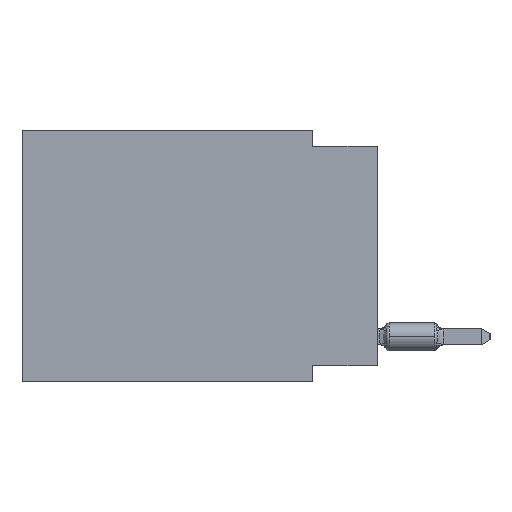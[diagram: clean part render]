
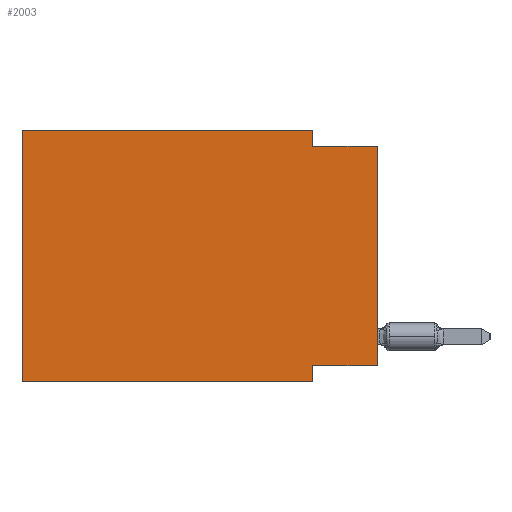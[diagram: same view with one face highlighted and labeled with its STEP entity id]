
A CAD part, left-side view. The second image highlights one B-rep face of the part: STEP entity #2003.
In plain terms, the highlighted planar face has unit normal (-1, 0, 0).
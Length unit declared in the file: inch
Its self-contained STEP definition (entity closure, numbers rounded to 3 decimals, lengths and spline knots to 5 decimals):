
#384 = PLANE ( 'NONE',  #32318 ) ;
#400 = LINE ( 'NONE', #17830, #42309 ) ;
#711 = VERTEX_POINT ( 'NONE', #39553 ) ;
#2003 = ADVANCED_FACE ( 'NONE', ( #34695 ), #384, .F. ) ;
#2099 = ORIENTED_EDGE ( 'NONE', *, *, #7044, .F. ) ;
#4460 = LINE ( 'NONE', #39086, #16757 ) ;
#5492 = CARTESIAN_POINT ( 'NONE',  ( 0., 0., -0.025 ) ) ;
#6367 = CARTESIAN_POINT ( 'NONE',  ( 0., 0.1, -0.39 ) ) ;
#7044 = EDGE_CURVE ( 'NONE', #51285, #8439, #31570, .T. ) ;
#8439 = VERTEX_POINT ( 'NONE', #15037 ) ;
#9232 = DIRECTION ( 'NONE',  ( 0., -1., 0. ) ) ;
#9585 = ORIENTED_EDGE ( 'NONE', *, *, #18488, .T. ) ;
#10608 = LINE ( 'NONE', #5492, #35398 ) ;
#12767 = LINE ( 'NONE', #21637, #32019 ) ;
#13049 = DIRECTION ( 'NONE',  ( 0., 1., 0. ) ) ;
#15013 = CARTESIAN_POINT ( 'NONE',  ( 0., 0.55, 0. ) ) ;
#15037 = CARTESIAN_POINT ( 'NONE',  ( 0., 0.1, -0.025 ) ) ;
#15389 = VERTEX_POINT ( 'NONE', #48682 ) ;
#16171 = VERTEX_POINT ( 'NONE', #43898 ) ;
#16757 = VECTOR ( 'NONE', #47970, 39.37008 ) ;
#17830 = CARTESIAN_POINT ( 'NONE',  ( 0., 0.55, -0.39 ) ) ;
#18095 = DIRECTION ( 'NONE',  ( 1., 0., 0. ) ) ;
#18488 = EDGE_CURVE ( 'NONE', #51190, #44938, #400, .T. ) ;
#18976 = EDGE_CURVE ( 'NONE', #711, #16171, #4460, .T. ) ;
#19512 = LINE ( 'NONE', #6367, #38303 ) ;
#21273 = ORIENTED_EDGE ( 'NONE', *, *, #32493, .F. ) ;
#21616 = CARTESIAN_POINT ( 'NONE',  ( 0., 0.55, 0. ) ) ;
#21637 = CARTESIAN_POINT ( 'NONE',  ( 0., 0., -0.365 ) ) ;
#21758 = EDGE_CURVE ( 'NONE', #51190, #42476, #39363, .T. ) ;
#23003 = DIRECTION ( 'NONE',  ( 0., 0., -1. ) ) ;
#23821 = DIRECTION ( 'NONE',  ( 0., 0., -1. ) ) ;
#25809 = CARTESIAN_POINT ( 'NONE',  ( 0., 0.55, 0. ) ) ;
#28436 = LINE ( 'NONE', #15013, #45415 ) ;
#29611 = ORIENTED_EDGE ( 'NONE', *, *, #18976, .T. ) ;
#31570 = LINE ( 'NONE', #49621, #54193 ) ;
#32019 = VECTOR ( 'NONE', #13049, 39.37008 ) ;
#32166 = ORIENTED_EDGE ( 'NONE', *, *, #43776, .F. ) ;
#32318 = AXIS2_PLACEMENT_3D ( 'NONE', #25809, #18095, #43866 ) ;
#32493 = EDGE_CURVE ( 'NONE', #15389, #44938, #19512, .T. ) ;
#34695 = FACE_OUTER_BOUND ( 'NONE', #53881, .T. ) ;
#35398 = VECTOR ( 'NONE', #54436, 39.37008 ) ;
#36012 = CARTESIAN_POINT ( 'NONE',  ( 0., 0.55, 0. ) ) ;
#36188 = DIRECTION ( 'NONE',  ( 0., -1., 0. ) ) ;
#36712 = CARTESIAN_POINT ( 'NONE',  ( 0., 0.55, -0.39 ) ) ;
#38303 = VECTOR ( 'NONE', #23821, 39.37008 ) ;
#39086 = CARTESIAN_POINT ( 'NONE',  ( 0., 0., 0. ) ) ;
#39363 = LINE ( 'NONE', #21616, #54457 ) ;
#39553 = CARTESIAN_POINT ( 'NONE',  ( 0., 0., -0.365 ) ) ;
#40119 = CARTESIAN_POINT ( 'NONE',  ( 0., 0.1, -0.39 ) ) ;
#41591 = CARTESIAN_POINT ( 'NONE',  ( 0., 0.1, 0. ) ) ;
#42309 = VECTOR ( 'NONE', #9232, 39.37008 ) ;
#42476 = VERTEX_POINT ( 'NONE', #36012 ) ;
#43094 = DIRECTION ( 'NONE',  ( 0., 0., 1. ) ) ;
#43776 = EDGE_CURVE ( 'NONE', #8439, #16171, #10608, .T. ) ;
#43866 = DIRECTION ( 'NONE',  ( 0., 0., -1. ) ) ;
#43898 = CARTESIAN_POINT ( 'NONE',  ( 0., 0., -0.025 ) ) ;
#44296 = ORIENTED_EDGE ( 'NONE', *, *, #53543, .F. ) ;
#44938 = VERTEX_POINT ( 'NONE', #40119 ) ;
#45415 = VECTOR ( 'NONE', #36188, 39.37008 ) ;
#47029 = EDGE_CURVE ( 'NONE', #42476, #51285, #28436, .T. ) ;
#47970 = DIRECTION ( 'NONE',  ( 0., 0., 1. ) ) ;
#48682 = CARTESIAN_POINT ( 'NONE',  ( 0., 0.1, -0.365 ) ) ;
#49621 = CARTESIAN_POINT ( 'NONE',  ( 0., 0.1, 0. ) ) ;
#50850 = ORIENTED_EDGE ( 'NONE', *, *, #21758, .F. ) ;
#51190 = VERTEX_POINT ( 'NONE', #36712 ) ;
#51285 = VERTEX_POINT ( 'NONE', #41591 ) ;
#53543 = EDGE_CURVE ( 'NONE', #711, #15389, #12767, .T. ) ;
#53881 = EDGE_LOOP ( 'NONE', ( #29611, #32166, #2099, #55707, #50850, #9585, #21273, #44296 ) ) ;
#54193 = VECTOR ( 'NONE', #23003, 39.37008 ) ;
#54436 = DIRECTION ( 'NONE',  ( 0., -1., 0. ) ) ;
#54457 = VECTOR ( 'NONE', #43094, 39.37008 ) ;
#55707 = ORIENTED_EDGE ( 'NONE', *, *, #47029, .F. ) ;
